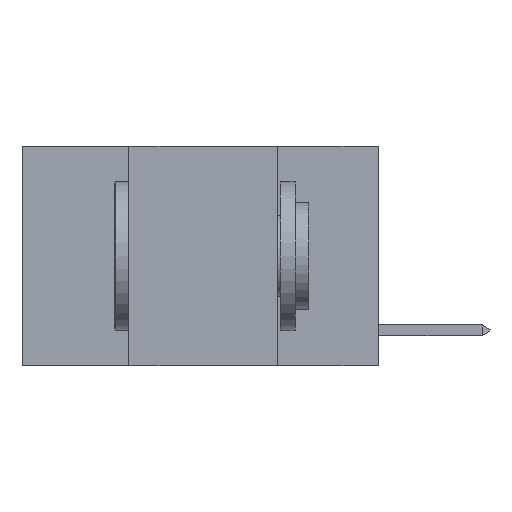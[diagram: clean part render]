
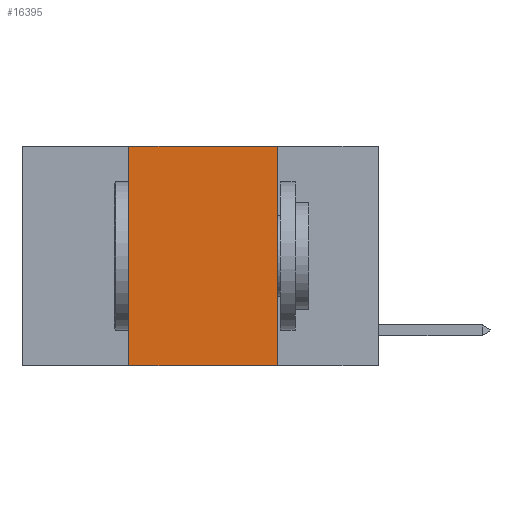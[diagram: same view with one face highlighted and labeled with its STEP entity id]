
A CAD part, left-side view. The second image highlights one B-rep face of the part: STEP entity #16395.
In plain terms, the highlighted planar face has unit normal (-1, 0, 0).
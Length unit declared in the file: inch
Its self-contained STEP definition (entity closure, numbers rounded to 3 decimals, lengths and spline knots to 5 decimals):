
#152 = ORIENTED_EDGE ( 'NONE', *, *, #17245, .T. ) ;
#1703 = EDGE_CURVE ( 'NONE', #1829, #2323, #13210, .T. ) ;
#1722 = EDGE_LOOP ( 'NONE', ( #7146, #5224, #17778, #152 ) ) ;
#1829 = VERTEX_POINT ( 'NONE', #8073 ) ;
#2145 = DIRECTION ( 'NONE',  ( 0., 0., 1. ) ) ;
#2282 = DIRECTION ( 'NONE',  ( 0., 0., -1. ) ) ;
#2323 = VERTEX_POINT ( 'NONE', #14548 ) ;
#3216 = VECTOR ( 'NONE', #2145, 39.37008 ) ;
#3837 = CARTESIAN_POINT ( 'NONE',  ( 0., 0.6, 0. ) ) ;
#5224 = ORIENTED_EDGE ( 'NONE', *, *, #17583, .F. ) ;
#5437 = LINE ( 'NONE', #9204, #17727 ) ;
#5630 = LINE ( 'NONE', #3837, #17086 ) ;
#6094 = CARTESIAN_POINT ( 'NONE',  ( 0., 0.17, 0. ) ) ;
#6311 = CARTESIAN_POINT ( 'NONE',  ( 0., 0.17, 0. ) ) ;
#7046 = DIRECTION ( 'NONE',  ( 0., 0., -1. ) ) ;
#7146 = ORIENTED_EDGE ( 'NONE', *, *, #20344, .F. ) ;
#8073 = CARTESIAN_POINT ( 'NONE',  ( 0., 0.42, -0.37 ) ) ;
#8687 = PLANE ( 'NONE',  #17038 ) ;
#9204 = CARTESIAN_POINT ( 'NONE',  ( 0., 0.6, -0.37 ) ) ;
#9511 = CARTESIAN_POINT ( 'NONE',  ( 0., 0.42, 0. ) ) ;
#11080 = VERTEX_POINT ( 'NONE', #6311 ) ;
#11086 = DIRECTION ( 'NONE',  ( 0., -1., 0. ) ) ;
#11624 = VECTOR ( 'NONE', #2282, 39.37008 ) ;
#11678 = LINE ( 'NONE', #6094, #11624 ) ;
#13210 = LINE ( 'NONE', #9511, #3216 ) ;
#14548 = CARTESIAN_POINT ( 'NONE',  ( 0., 0.42, 0. ) ) ;
#14601 = DIRECTION ( 'NONE',  ( 0., -1., 0. ) ) ;
#15806 = CARTESIAN_POINT ( 'NONE',  ( 0., 0.17, -0.37 ) ) ;
#15985 = CARTESIAN_POINT ( 'NONE',  ( 0., 0.6, 0. ) ) ;
#16395 = ADVANCED_FACE ( 'NONE', ( #17783 ), #8687, .F. ) ;
#17038 = AXIS2_PLACEMENT_3D ( 'NONE', #15985, #23235, #7046 ) ;
#17086 = VECTOR ( 'NONE', #11086, 39.37008 ) ;
#17245 = EDGE_CURVE ( 'NONE', #1829, #21253, #5437, .T. ) ;
#17583 = EDGE_CURVE ( 'NONE', #2323, #11080, #5630, .T. ) ;
#17727 = VECTOR ( 'NONE', #14601, 39.37008 ) ;
#17778 = ORIENTED_EDGE ( 'NONE', *, *, #1703, .F. ) ;
#17783 = FACE_OUTER_BOUND ( 'NONE', #1722, .T. ) ;
#20344 = EDGE_CURVE ( 'NONE', #11080, #21253, #11678, .T. ) ;
#21253 = VERTEX_POINT ( 'NONE', #15806 ) ;
#23235 = DIRECTION ( 'NONE',  ( 1., 0., 0. ) ) ;
